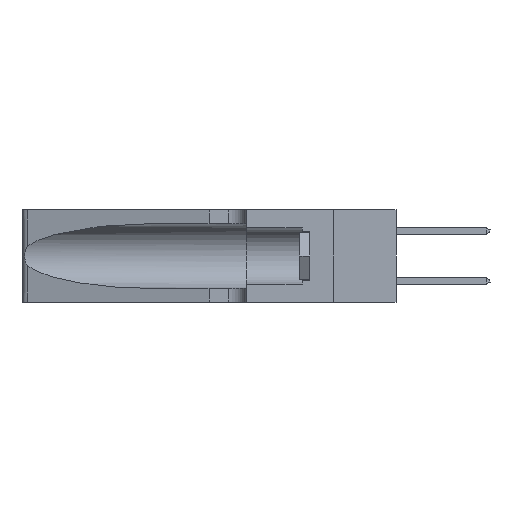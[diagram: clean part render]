
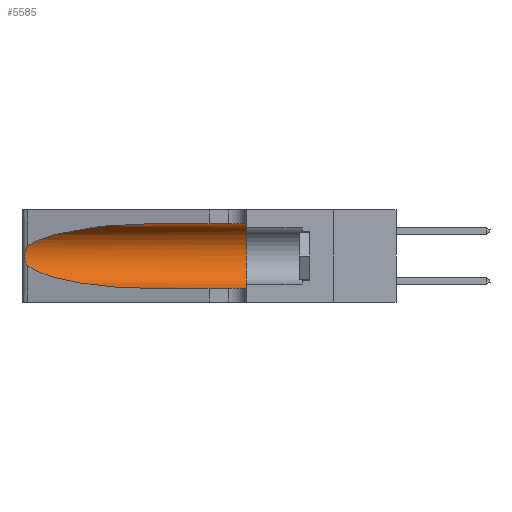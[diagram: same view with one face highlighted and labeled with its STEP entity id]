
A CAD part, left-side view. The second image highlights one B-rep face of the part: STEP entity #5585.
In plain terms, the highlighted cylindrical face has radius 3.308 mm (diameter 6.617 mm), a partial arc.
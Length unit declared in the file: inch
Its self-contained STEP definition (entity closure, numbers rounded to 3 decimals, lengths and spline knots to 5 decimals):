
#35 = CARTESIAN_POINT ( 'NONE',  ( 0.25487, 1.22718, 0.14631 ) ) ;
#424 = DIRECTION ( 'NONE',  ( 0., 0., -1. ) ) ;
#936 = CARTESIAN_POINT ( 'NONE',  ( 0.1305, 0.35, 0.05475 ) ) ;
#1204 = CARTESIAN_POINT ( 'NONE',  ( 0.26075, 1.23896, 0.19203 ) ) ;
#1363 = CARTESIAN_POINT ( 'NONE',  ( 0.1305, 0.72297, 0.31525 ) ) ;
#1895 = EDGE_CURVE ( 'NONE', #7969, #11842, #19501, .T. ) ;
#2439 = ORIENTED_EDGE ( 'NONE', *, *, #14707, .T. ) ;
#2481 = AXIS2_PLACEMENT_3D ( 'NONE', #18271, #8683, #10278 ) ;
#2580 = EDGE_CURVE ( 'NONE', #11842, #13588, #17956, .T. ) ;
#2855 = CARTESIAN_POINT ( 'NONE',  ( 0.1305, 1.61858, 0.31525 ) ) ;
#2909 = CARTESIAN_POINT ( 'NONE',  ( 0.2373, 1.15595, 0.28018 ) ) ;
#3296 = VERTEX_POINT ( 'NONE', #7197 ) ;
#3563 = LINE ( 'NONE', #16318, #4058 ) ;
#4058 = VECTOR ( 'NONE', #20332, 39.37008 ) ;
#4434 = CARTESIAN_POINT ( 'NONE',  ( 0.1305, 0.72297, 0.05475 ) ) ;
#5585 = ADVANCED_FACE ( 'NONE', ( #19969 ), #15176, .F. ) ;
#6086 = CARTESIAN_POINT ( 'NONE',  ( 0.25639, 1.23186, 0.15144 ) ) ;
#6562 = CARTESIAN_POINT ( 'NONE',  ( 0.26018, 1.23835, 0.19895 ) ) ;
#6647 = EDGE_CURVE ( 'NONE', #11024, #13588, #3563, .T. ) ;
#7197 = CARTESIAN_POINT ( 'NONE',  ( 0.25487, 1.22718, 0.22369 ) ) ;
#7574 = CARTESIAN_POINT ( 'NONE',  ( 0.26017, 1.23833, 0.17102 ) ) ;
#7591 = DIRECTION ( 'NONE',  ( 0., -1., 0. ) ) ;
#7599 = CARTESIAN_POINT ( 'NONE',  ( 0.25639, 1.23184, 0.21858 ) ) ;
#7861 = CARTESIAN_POINT ( 'NONE',  ( 0.25789, 1.23486, 0.15765 ) ) ;
#7969 = VERTEX_POINT ( 'NONE', #16612 ) ;
#8158 = CARTESIAN_POINT ( 'NONE',  ( 0.18966, 0.96281, 0.31525 ) ) ;
#8228 = EDGE_LOOP ( 'NONE', ( #2439, #10987, #15364, #19844, #15068, #12737 ) ) ;
#8350 = CARTESIAN_POINT ( 'NONE',  ( 0.1305, 0.72297, 0.05475 ) ) ;
#8611 = CARTESIAN_POINT ( 'NONE',  ( 0.25555, 1.22993, 0.14849 ) ) ;
#8683 = DIRECTION ( 'NONE',  ( 0., 1., 0. ) ) ;
#9367 = CARTESIAN_POINT ( 'NONE',  ( 0.25555, 1.22994, 0.2215 ) ) ;
#9462 = CARTESIAN_POINT ( 'NONE',  ( 0.25787, 1.23484, 0.2124 ) ) ;
#10278 = DIRECTION ( 'NONE',  ( 0., 0., 1. ) ) ;
#10479 = CARTESIAN_POINT ( 'NONE',  ( 0.1305, 0.35, 0.31525 ) ) ;
#10987 = ORIENTED_EDGE ( 'NONE', *, *, #14470, .T. ) ;
#11024 = VERTEX_POINT ( 'NONE', #4434 ) ;
#11397 = CARTESIAN_POINT ( 'NONE',  ( 0.25487, 1.22718, 0.14631 ) ) ;
#11538 = CARTESIAN_POINT ( 'NONE',  ( 0.25487, 1.22718, 0.14631 ) ) ;
#11842 = VERTEX_POINT ( 'NONE', #10479 ) ;
#12549 = CARTESIAN_POINT ( 'NONE',  ( 0.25487, 1.22718, 0.22369 ) ) ;
#12651 =( BOUNDED_CURVE ( )  B_SPLINE_CURVE ( 3, ( #35, #16186, #19587, #8350 ),
 .UNSPECIFIED., .F., .F. ) 
 B_SPLINE_CURVE_WITH_KNOTS ( ( 4, 4 ),
 ( 3.44316, 4.71239 ),
 .UNSPECIFIED. ) 
 CURVE ( )  GEOMETRIC_REPRESENTATION_ITEM ( )  RATIONAL_B_SPLINE_CURVE ( ( 1., 0.87, 0.87, 1. ) ) 
 REPRESENTATION_ITEM ( '' )  );
#12737 = ORIENTED_EDGE ( 'NONE', *, *, #1895, .F. ) ;
#12808 = CARTESIAN_POINT ( 'NONE',  ( 0.1305, 1.61858, 0.185 ) ) ;
#13204 = VECTOR ( 'NONE', #18828, 39.37008 ) ;
#13588 = VERTEX_POINT ( 'NONE', #936 ) ;
#14470 = EDGE_CURVE ( 'NONE', #3296, #15493, #20106, .T. ) ;
#14707 = EDGE_CURVE ( 'NONE', #7969, #3296, #16383, .T. ) ;
#15068 = ORIENTED_EDGE ( 'NONE', *, *, #2580, .F. ) ;
#15176 = CYLINDRICAL_SURFACE ( 'NONE', #20090, 0.13025 ) ;
#15364 = ORIENTED_EDGE ( 'NONE', *, *, #18768, .T. ) ;
#15493 = VERTEX_POINT ( 'NONE', #11397 ) ;
#16186 = CARTESIAN_POINT ( 'NONE',  ( 0.2373, 1.15595, 0.08982 ) ) ;
#16318 = CARTESIAN_POINT ( 'NONE',  ( 0.1305, 1.61858, 0.05475 ) ) ;
#16383 =( BOUNDED_CURVE ( )  B_SPLINE_CURVE ( 3, ( #1363, #8158, #2909, #12549 ),
 .UNSPECIFIED., .F., .F. ) 
 B_SPLINE_CURVE_WITH_KNOTS ( ( 4, 4 ),
 ( 1.5708, 2.84003 ),
 .UNSPECIFIED. ) 
 CURVE ( )  GEOMETRIC_REPRESENTATION_ITEM ( )  RATIONAL_B_SPLINE_CURVE ( ( 1., 0.87, 0.87, 1. ) ) 
 REPRESENTATION_ITEM ( '' )  );
#16450 = CARTESIAN_POINT ( 'NONE',  ( 0.25487, 1.22718, 0.22369 ) ) ;
#16612 = CARTESIAN_POINT ( 'NONE',  ( 0.1305, 0.72297, 0.31525 ) ) ;
#17956 = CIRCLE ( 'NONE', #2481, 0.13025 ) ;
#18271 = CARTESIAN_POINT ( 'NONE',  ( 0.1305, 0.35, 0.185 ) ) ;
#18768 = EDGE_CURVE ( 'NONE', #15493, #11024, #12651, .T. ) ;
#18828 = DIRECTION ( 'NONE',  ( 0., -1., 0. ) ) ;
#19024 = CARTESIAN_POINT ( 'NONE',  ( 0.25856, 1.23593, 0.16098 ) ) ;
#19501 = LINE ( 'NONE', #2855, #13204 ) ;
#19587 = CARTESIAN_POINT ( 'NONE',  ( 0.18966, 0.96281, 0.05475 ) ) ;
#19844 = ORIENTED_EDGE ( 'NONE', *, *, #6647, .T. ) ;
#19969 = FACE_OUTER_BOUND ( 'NONE', #8228, .T. ) ;
#20090 = AXIS2_PLACEMENT_3D ( 'NONE', #12808, #7591, #424 ) ;
#20106 = B_SPLINE_CURVE_WITH_KNOTS ( 'NONE', 3,
 ( #16450, #9367, #7599, #9462, #20349, #6562, #1204, #20485, #7574, #19024, #7861, #6086, #8611, #11538 ),
 .UNSPECIFIED., .F., .F.,
 ( 4, 2, 2, 2, 2, 2, 4 ),
 ( 0., 0.00027, 0.00053, 0.00107, 0.0016, 0.00187, 0.00214 ),
 .UNSPECIFIED. ) ;
#20332 = DIRECTION ( 'NONE',  ( 0., -1., 0. ) ) ;
#20349 = CARTESIAN_POINT ( 'NONE',  ( 0.25854, 1.2359, 0.20912 ) ) ;
#20485 = CARTESIAN_POINT ( 'NONE',  ( 0.26075, 1.23896, 0.178 ) ) ;
